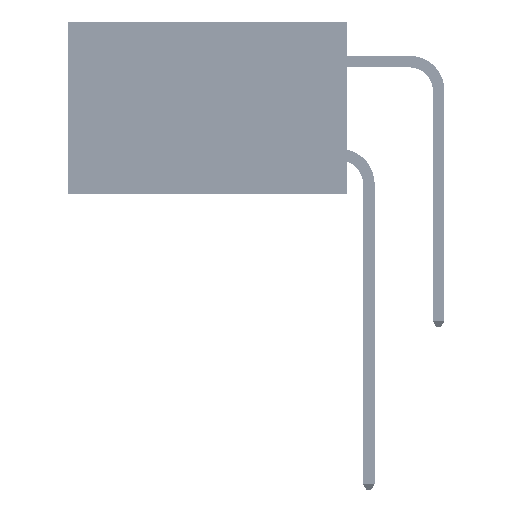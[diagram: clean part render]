
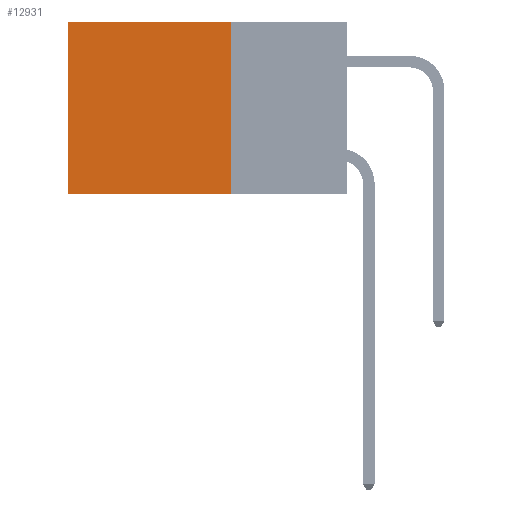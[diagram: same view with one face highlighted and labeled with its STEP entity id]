
A CAD part, left-side view. The second image highlights one B-rep face of the part: STEP entity #12931.
In plain terms, the highlighted planar face has unit normal (-1, 0, 0).
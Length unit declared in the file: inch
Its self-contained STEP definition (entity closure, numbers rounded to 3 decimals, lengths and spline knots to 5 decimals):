
#247 = EDGE_CURVE ( 'NONE', #5610, #25441, #9329, .T. ) ;
#1654 = CARTESIAN_POINT ( 'NONE',  ( 0.2875, 0.25, 0. ) ) ;
#2776 = DIRECTION ( 'NONE',  ( 0., 0., -1. ) ) ;
#4982 = VERTEX_POINT ( 'NONE', #31647 ) ;
#5610 = VERTEX_POINT ( 'NONE', #1654 ) ;
#6311 = EDGE_CURVE ( 'NONE', #53058, #4982, #26170, .T. ) ;
#9259 = VECTOR ( 'NONE', #26953, 39.37008 ) ;
#9329 = LINE ( 'NONE', #38995, #17796 ) ;
#9819 = ORIENTED_EDGE ( 'NONE', *, *, #21082, .T. ) ;
#11189 = LINE ( 'NONE', #14379, #9259 ) ;
#11555 = PLANE ( 'NONE',  #15058 ) ;
#12931 = ADVANCED_FACE ( 'NONE', ( #29551 ), #11555, .F. ) ;
#14379 = CARTESIAN_POINT ( 'NONE',  ( 0.2875, 0.25, 0. ) ) ;
#15058 = AXIS2_PLACEMENT_3D ( 'NONE', #19930, #28692, #15911 ) ;
#15911 = DIRECTION ( 'NONE',  ( 0., 0., -1. ) ) ;
#16157 = LINE ( 'NONE', #48105, #46901 ) ;
#17796 = VECTOR ( 'NONE', #30229, 39.37008 ) ;
#19104 = EDGE_CURVE ( 'NONE', #5610, #53058, #11189, .T. ) ;
#19930 = CARTESIAN_POINT ( 'NONE',  ( 0.2875, 0.25, 0. ) ) ;
#21082 = EDGE_CURVE ( 'NONE', #25441, #4982, #16157, .T. ) ;
#21260 = ORIENTED_EDGE ( 'NONE', *, *, #6311, .F. ) ;
#25441 = VERTEX_POINT ( 'NONE', #27428 ) ;
#26170 = LINE ( 'NONE', #39556, #30101 ) ;
#26953 = DIRECTION ( 'NONE',  ( 0., 0., -1. ) ) ;
#27428 = CARTESIAN_POINT ( 'NONE',  ( 0.2875, 0.6, 0. ) ) ;
#28692 = DIRECTION ( 'NONE',  ( 1., 0., 0. ) ) ;
#29551 = FACE_OUTER_BOUND ( 'NONE', #49366, .T. ) ;
#29886 = ORIENTED_EDGE ( 'NONE', *, *, #19104, .F. ) ;
#30101 = VECTOR ( 'NONE', #47424, 39.37008 ) ;
#30229 = DIRECTION ( 'NONE',  ( 0., 1., 0. ) ) ;
#31647 = CARTESIAN_POINT ( 'NONE',  ( 0.2875, 0.6, -0.37 ) ) ;
#38995 = CARTESIAN_POINT ( 'NONE',  ( 0.2875, 0.25, 0. ) ) ;
#39556 = CARTESIAN_POINT ( 'NONE',  ( 0.2875, 0.25, -0.37 ) ) ;
#40605 = CARTESIAN_POINT ( 'NONE',  ( 0.2875, 0.25, -0.37 ) ) ;
#42449 = ORIENTED_EDGE ( 'NONE', *, *, #247, .T. ) ;
#46901 = VECTOR ( 'NONE', #2776, 39.37008 ) ;
#47424 = DIRECTION ( 'NONE',  ( 0., 1., 0. ) ) ;
#48105 = CARTESIAN_POINT ( 'NONE',  ( 0.2875, 0.6, 0. ) ) ;
#49366 = EDGE_LOOP ( 'NONE', ( #9819, #21260, #29886, #42449 ) ) ;
#53058 = VERTEX_POINT ( 'NONE', #40605 ) ;
